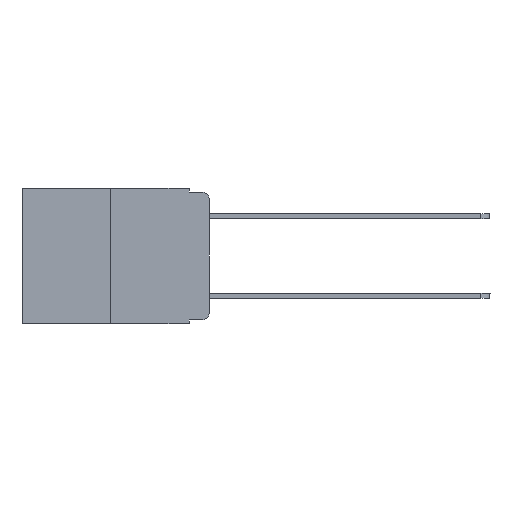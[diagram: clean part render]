
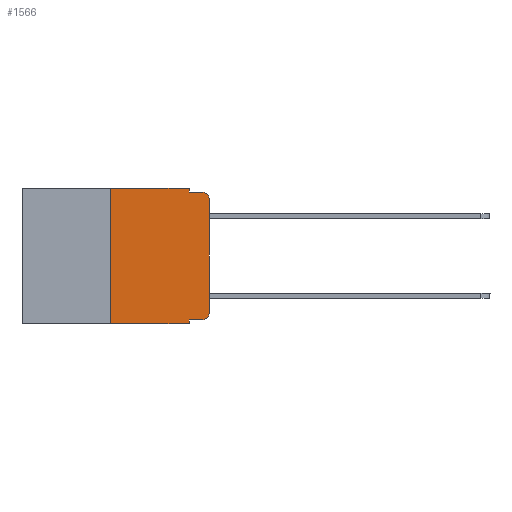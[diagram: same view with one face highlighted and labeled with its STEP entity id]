
A CAD part, left-side view. The second image highlights one B-rep face of the part: STEP entity #1566.
In plain terms, the highlighted planar face has unit normal (-1, 0, 0).
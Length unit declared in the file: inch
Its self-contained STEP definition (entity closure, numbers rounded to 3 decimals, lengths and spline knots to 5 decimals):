
#124 = CARTESIAN_POINT ( 'NONE',  ( 0., 0.02, -0.01 ) ) ;
#253 = CARTESIAN_POINT ( 'NONE',  ( 0., 0.051, 0. ) ) ;
#445 = ORIENTED_EDGE ( 'NONE', *, *, #6201, .T. ) ;
#507 = CARTESIAN_POINT ( 'NONE',  ( 0., 0., 0. ) ) ;
#652 = EDGE_CURVE ( 'NONE', #10101, #9031, #9509, .T. ) ;
#749 = CARTESIAN_POINT ( 'NONE',  ( 0., 0.473, -0.343 ) ) ;
#798 = DIRECTION ( 'NONE',  ( -1., 0., 0. ) ) ;
#866 = VERTEX_POINT ( 'NONE', #5719 ) ;
#1066 = CARTESIAN_POINT ( 'NONE',  ( 0., 0.25, 0. ) ) ;
#1106 = LINE ( 'NONE', #3786, #10139 ) ;
#1256 = CIRCLE ( 'NONE', #3525, 0.02 ) ;
#1299 = CIRCLE ( 'NONE', #8104, 0.02 ) ;
#1329 = DIRECTION ( 'NONE',  ( 0., -1., 0. ) ) ;
#1475 = LINE ( 'NONE', #749, #7787 ) ;
#1480 = EDGE_LOOP ( 'NONE', ( #4450, #445, #3072, #9181, #4916, #2226, #3437, #7277, #10321, #3966 ) ) ;
#1487 = VECTOR ( 'NONE', #3988, 39.37008 ) ;
#1566 = ADVANCED_FACE ( 'NONE', ( #5819 ), #6124, .F. ) ;
#2006 = VECTOR ( 'NONE', #2729, 39.37008 ) ;
#2221 = CARTESIAN_POINT ( 'NONE',  ( 0., 0., -0.03 ) ) ;
#2226 = ORIENTED_EDGE ( 'NONE', *, *, #7650, .F. ) ;
#2428 = EDGE_CURVE ( 'NONE', #4937, #6764, #10690, .T. ) ;
#2513 = DIRECTION ( 'NONE',  ( 0., 0., -1. ) ) ;
#2663 = CARTESIAN_POINT ( 'NONE',  ( 0., 0.25, -0.343 ) ) ;
#2729 = DIRECTION ( 'NONE',  ( 0., 0., 1. ) ) ;
#2878 = VECTOR ( 'NONE', #4647, 39.37008 ) ;
#2900 = DIRECTION ( 'NONE',  ( 0., -1., 0. ) ) ;
#3001 = CARTESIAN_POINT ( 'NONE',  ( 0., 0.051, 0. ) ) ;
#3072 = ORIENTED_EDGE ( 'NONE', *, *, #652, .F. ) ;
#3377 = AXIS2_PLACEMENT_3D ( 'NONE', #9539, #4311, #4472 ) ;
#3437 = ORIENTED_EDGE ( 'NONE', *, *, #5001, .T. ) ;
#3525 = AXIS2_PLACEMENT_3D ( 'NONE', #7047, #5284, #2513 ) ;
#3786 = CARTESIAN_POINT ( 'NONE',  ( 0., 0.473, 0. ) ) ;
#3966 = ORIENTED_EDGE ( 'NONE', *, *, #10254, .T. ) ;
#3988 = DIRECTION ( 'NONE',  ( 0., 0., 1. ) ) ;
#4101 = LINE ( 'NONE', #507, #1487 ) ;
#4198 = EDGE_CURVE ( 'NONE', #10916, #10101, #9285, .T. ) ;
#4239 = DIRECTION ( 'NONE',  ( 0., -1., 0. ) ) ;
#4311 = DIRECTION ( 'NONE',  ( 1., 0., 0. ) ) ;
#4406 = EDGE_CURVE ( 'NONE', #866, #5502, #4101, .T. ) ;
#4450 = ORIENTED_EDGE ( 'NONE', *, *, #4406, .T. ) ;
#4472 = DIRECTION ( 'NONE',  ( 0., 0., -1. ) ) ;
#4647 = DIRECTION ( 'NONE',  ( 0., 0., -1. ) ) ;
#4916 = ORIENTED_EDGE ( 'NONE', *, *, #10464, .F. ) ;
#4937 = VERTEX_POINT ( 'NONE', #5717 ) ;
#5001 = EDGE_CURVE ( 'NONE', #6712, #6764, #1475, .T. ) ;
#5187 = CARTESIAN_POINT ( 'NONE',  ( 0., 0.02, -0.333 ) ) ;
#5269 = CARTESIAN_POINT ( 'NONE',  ( 0., 0.051, -0.01 ) ) ;
#5284 = DIRECTION ( 'NONE',  ( -1., 0., 0. ) ) ;
#5392 = DIRECTION ( 'NONE',  ( 0., 0., -1. ) ) ;
#5502 = VERTEX_POINT ( 'NONE', #2221 ) ;
#5717 = CARTESIAN_POINT ( 'NONE',  ( 0., 0.051, -0.333 ) ) ;
#5719 = CARTESIAN_POINT ( 'NONE',  ( 0., 0., -0.313 ) ) ;
#5819 = FACE_OUTER_BOUND ( 'NONE', #1480, .T. ) ;
#5824 = CARTESIAN_POINT ( 'NONE',  ( 0., 0.051, -0.01 ) ) ;
#6124 = PLANE ( 'NONE',  #3377 ) ;
#6201 = EDGE_CURVE ( 'NONE', #5502, #9031, #1299, .T. ) ;
#6246 = CARTESIAN_POINT ( 'NONE',  ( 0., 0.051, -0.343 ) ) ;
#6264 = VECTOR ( 'NONE', #1329, 39.37008 ) ;
#6375 = EDGE_CURVE ( 'NONE', #4937, #8041, #9104, .T. ) ;
#6388 = CARTESIAN_POINT ( 'NONE',  ( 0., 0.051, 0. ) ) ;
#6600 = CARTESIAN_POINT ( 'NONE',  ( 0., 0.051, -0.333 ) ) ;
#6631 = VECTOR ( 'NONE', #5392, 39.37008 ) ;
#6712 = VERTEX_POINT ( 'NONE', #2663 ) ;
#6764 = VERTEX_POINT ( 'NONE', #6246 ) ;
#7047 = CARTESIAN_POINT ( 'NONE',  ( 0., 0.02, -0.313 ) ) ;
#7277 = ORIENTED_EDGE ( 'NONE', *, *, #2428, .F. ) ;
#7650 = EDGE_CURVE ( 'NONE', #6712, #7869, #9543, .T. ) ;
#7787 = VECTOR ( 'NONE', #4239, 39.37008 ) ;
#7869 = VERTEX_POINT ( 'NONE', #1066 ) ;
#8041 = VERTEX_POINT ( 'NONE', #5187 ) ;
#8104 = AXIS2_PLACEMENT_3D ( 'NONE', #10376, #798, #9553 ) ;
#9031 = VERTEX_POINT ( 'NONE', #124 ) ;
#9104 = LINE ( 'NONE', #6600, #6264 ) ;
#9181 = ORIENTED_EDGE ( 'NONE', *, *, #4198, .F. ) ;
#9285 = LINE ( 'NONE', #253, #2878 ) ;
#9509 = LINE ( 'NONE', #5269, #10871 ) ;
#9539 = CARTESIAN_POINT ( 'NONE',  ( 0., 0.473, 0. ) ) ;
#9543 = LINE ( 'NONE', #9634, #2006 ) ;
#9553 = DIRECTION ( 'NONE',  ( 0., 0., -1. ) ) ;
#9634 = CARTESIAN_POINT ( 'NONE',  ( 0., 0.25, 0. ) ) ;
#10101 = VERTEX_POINT ( 'NONE', #5824 ) ;
#10139 = VECTOR ( 'NONE', #2900, 39.37008 ) ;
#10254 = EDGE_CURVE ( 'NONE', #8041, #866, #1256, .T. ) ;
#10321 = ORIENTED_EDGE ( 'NONE', *, *, #6375, .T. ) ;
#10376 = CARTESIAN_POINT ( 'NONE',  ( 0., 0.02, -0.03 ) ) ;
#10464 = EDGE_CURVE ( 'NONE', #7869, #10916, #1106, .T. ) ;
#10509 = DIRECTION ( 'NONE',  ( 0., -1., 0. ) ) ;
#10690 = LINE ( 'NONE', #6388, #6631 ) ;
#10871 = VECTOR ( 'NONE', #10509, 39.37008 ) ;
#10916 = VERTEX_POINT ( 'NONE', #3001 ) ;
